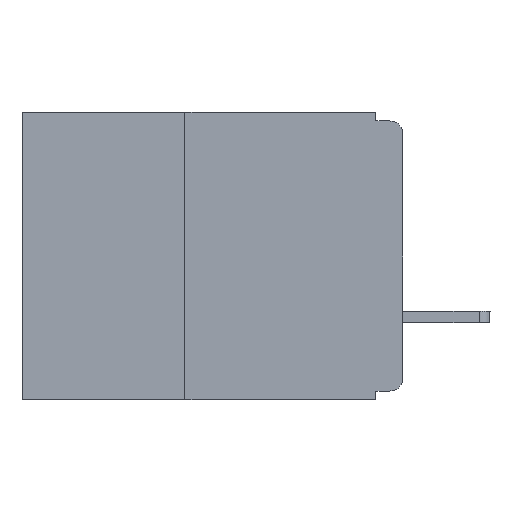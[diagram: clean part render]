
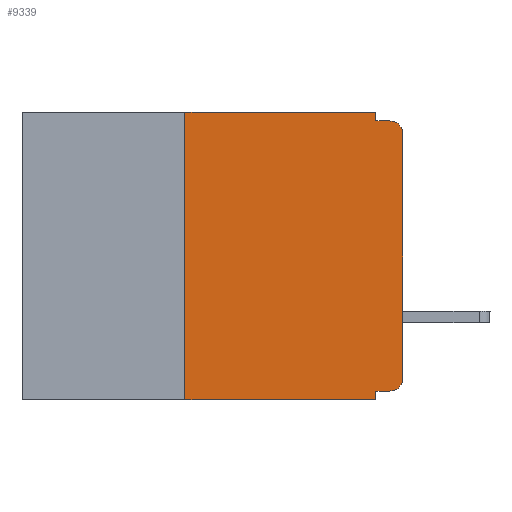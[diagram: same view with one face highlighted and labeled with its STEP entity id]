
A CAD part, left-side view. The second image highlights one B-rep face of the part: STEP entity #9339.
In plain terms, the highlighted planar face has unit normal (-1, 0, 0).
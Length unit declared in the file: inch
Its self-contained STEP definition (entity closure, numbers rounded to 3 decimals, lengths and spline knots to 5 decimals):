
#424 = CARTESIAN_POINT ( 'NONE',  ( 0., 0.015, -0.01 ) ) ;
#497 = EDGE_CURVE ( 'NONE', #14240, #14907, #5640, .T. ) ;
#506 = DIRECTION ( 'NONE',  ( 0., 1., 0. ) ) ;
#738 = ORIENTED_EDGE ( 'NONE', *, *, #2912, .F. ) ;
#810 = EDGE_CURVE ( 'NONE', #11780, #13510, #9364, .T. ) ;
#828 = CARTESIAN_POINT ( 'NONE',  ( 0., 0.25, 0. ) ) ;
#1467 = LINE ( 'NONE', #8580, #14368 ) ;
#1536 = CARTESIAN_POINT ( 'NONE',  ( 0., 0.437, 0. ) ) ;
#2530 = VERTEX_POINT ( 'NONE', #14855 ) ;
#2590 = EDGE_CURVE ( 'NONE', #13633, #3696, #1467, .T. ) ;
#2647 = CARTESIAN_POINT ( 'NONE',  ( 0., 0.031, -0.33 ) ) ;
#2655 = DIRECTION ( 'NONE',  ( 0., 0., -1. ) ) ;
#2823 = DIRECTION ( 'NONE',  ( 0., 0., -1. ) ) ;
#2912 = EDGE_CURVE ( 'NONE', #3696, #2530, #3793, .T. ) ;
#3061 = VERTEX_POINT ( 'NONE', #424 ) ;
#3196 = DIRECTION ( 'NONE',  ( 0., 0., 1. ) ) ;
#3509 = ORIENTED_EDGE ( 'NONE', *, *, #4165, .F. ) ;
#3512 = CARTESIAN_POINT ( 'NONE',  ( 0., 0.25, -0.33 ) ) ;
#3549 = LINE ( 'NONE', #13216, #4537 ) ;
#3696 = VERTEX_POINT ( 'NONE', #7413 ) ;
#3706 = CARTESIAN_POINT ( 'NONE',  ( 0., 0.25, -0.33 ) ) ;
#3776 = VECTOR ( 'NONE', #11013, 39.37008 ) ;
#3793 = LINE ( 'NONE', #15214, #13021 ) ;
#3860 = CARTESIAN_POINT ( 'NONE',  ( 0., 0.031, -0.33 ) ) ;
#4006 = AXIS2_PLACEMENT_3D ( 'NONE', #1536, #10314, #15350 ) ;
#4069 = ORIENTED_EDGE ( 'NONE', *, *, #8922, .T. ) ;
#4165 = EDGE_CURVE ( 'NONE', #14240, #13633, #4741, .T. ) ;
#4209 = VECTOR ( 'NONE', #506, 39.37008 ) ;
#4396 = DIRECTION ( 'NONE',  ( 0., -1., 0. ) ) ;
#4537 = VECTOR ( 'NONE', #3196, 39.37008 ) ;
#4741 = LINE ( 'NONE', #3706, #14886 ) ;
#5272 = PLANE ( 'NONE',  #4006 ) ;
#5459 = CARTESIAN_POINT ( 'NONE',  ( 0., 0.015, -0.305 ) ) ;
#5632 = DIRECTION ( 'NONE',  ( -1., 0., 0. ) ) ;
#5640 = LINE ( 'NONE', #10666, #8775 ) ;
#5997 = VERTEX_POINT ( 'NONE', #9700 ) ;
#6373 = CARTESIAN_POINT ( 'NONE',  ( 0., 0.015, -0.025 ) ) ;
#7054 = AXIS2_PLACEMENT_3D ( 'NONE', #5459, #5632, #9283 ) ;
#7408 = EDGE_CURVE ( 'NONE', #2530, #3061, #14342, .T. ) ;
#7413 = CARTESIAN_POINT ( 'NONE',  ( 0., 0.031, 0. ) ) ;
#7627 = EDGE_CURVE ( 'NONE', #5997, #14907, #10260, .T. ) ;
#8301 = ORIENTED_EDGE ( 'NONE', *, *, #7408, .F. ) ;
#8580 = CARTESIAN_POINT ( 'NONE',  ( 0., 0.437, 0. ) ) ;
#8707 = DIRECTION ( 'NONE',  ( 0., 0., 1. ) ) ;
#8735 = EDGE_CURVE ( 'NONE', #8907, #3061, #10041, .T. ) ;
#8775 = VECTOR ( 'NONE', #4396, 39.37008 ) ;
#8907 = VERTEX_POINT ( 'NONE', #9603 ) ;
#8922 = EDGE_CURVE ( 'NONE', #13510, #8907, #3549, .T. ) ;
#9283 = DIRECTION ( 'NONE',  ( 0., 0., -1. ) ) ;
#9327 = ORIENTED_EDGE ( 'NONE', *, *, #497, .T. ) ;
#9339 = ADVANCED_FACE ( 'NONE', ( #13148 ), #5272, .F. ) ;
#9364 = CIRCLE ( 'NONE', #7054, 0.015 ) ;
#9603 = CARTESIAN_POINT ( 'NONE',  ( 0., 0., -0.025 ) ) ;
#9700 = CARTESIAN_POINT ( 'NONE',  ( 0., 0.031, -0.32 ) ) ;
#9824 = EDGE_LOOP ( 'NONE', ( #4069, #15046, #8301, #738, #12819, #3509, #9327, #10227, #9886, #12751 ) ) ;
#9886 = ORIENTED_EDGE ( 'NONE', *, *, #15507, .F. ) ;
#10002 = AXIS2_PLACEMENT_3D ( 'NONE', #6373, #15152, #2655 ) ;
#10041 = CIRCLE ( 'NONE', #10002, 0.015 ) ;
#10227 = ORIENTED_EDGE ( 'NONE', *, *, #7627, .F. ) ;
#10260 = LINE ( 'NONE', #2647, #12609 ) ;
#10314 = DIRECTION ( 'NONE',  ( 1., 0., 0. ) ) ;
#10422 = CARTESIAN_POINT ( 'NONE',  ( 0., 0.015, -0.32 ) ) ;
#10499 = DIRECTION ( 'NONE',  ( 0., 0., -1. ) ) ;
#10666 = CARTESIAN_POINT ( 'NONE',  ( 0., 0.437, -0.33 ) ) ;
#11013 = DIRECTION ( 'NONE',  ( 0., -1., 0. ) ) ;
#11780 = VERTEX_POINT ( 'NONE', #10422 ) ;
#11965 = CARTESIAN_POINT ( 'NONE',  ( 0., 0., -0.305 ) ) ;
#12268 = CARTESIAN_POINT ( 'NONE',  ( 0., 0., -0.01 ) ) ;
#12609 = VECTOR ( 'NONE', #10499, 39.37008 ) ;
#12751 = ORIENTED_EDGE ( 'NONE', *, *, #810, .T. ) ;
#12819 = ORIENTED_EDGE ( 'NONE', *, *, #2590, .F. ) ;
#13021 = VECTOR ( 'NONE', #2823, 39.37008 ) ;
#13148 = FACE_OUTER_BOUND ( 'NONE', #9824, .T. ) ;
#13150 = CARTESIAN_POINT ( 'NONE',  ( 0., 0., -0.32 ) ) ;
#13216 = CARTESIAN_POINT ( 'NONE',  ( 0., 0., 0. ) ) ;
#13510 = VERTEX_POINT ( 'NONE', #11965 ) ;
#13613 = LINE ( 'NONE', #13150, #4209 ) ;
#13633 = VERTEX_POINT ( 'NONE', #828 ) ;
#14240 = VERTEX_POINT ( 'NONE', #3512 ) ;
#14342 = LINE ( 'NONE', #12268, #3776 ) ;
#14368 = VECTOR ( 'NONE', #14784, 39.37008 ) ;
#14784 = DIRECTION ( 'NONE',  ( 0., -1., 0. ) ) ;
#14855 = CARTESIAN_POINT ( 'NONE',  ( 0., 0.031, -0.01 ) ) ;
#14886 = VECTOR ( 'NONE', #8707, 39.37008 ) ;
#14907 = VERTEX_POINT ( 'NONE', #3860 ) ;
#15046 = ORIENTED_EDGE ( 'NONE', *, *, #8735, .T. ) ;
#15152 = DIRECTION ( 'NONE',  ( -1., 0., 0. ) ) ;
#15214 = CARTESIAN_POINT ( 'NONE',  ( 0., 0.031, 0. ) ) ;
#15350 = DIRECTION ( 'NONE',  ( 0., 0., -1. ) ) ;
#15507 = EDGE_CURVE ( 'NONE', #11780, #5997, #13613, .T. ) ;
